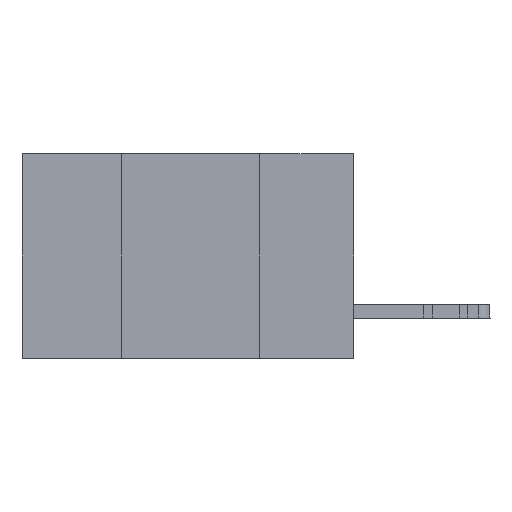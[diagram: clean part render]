
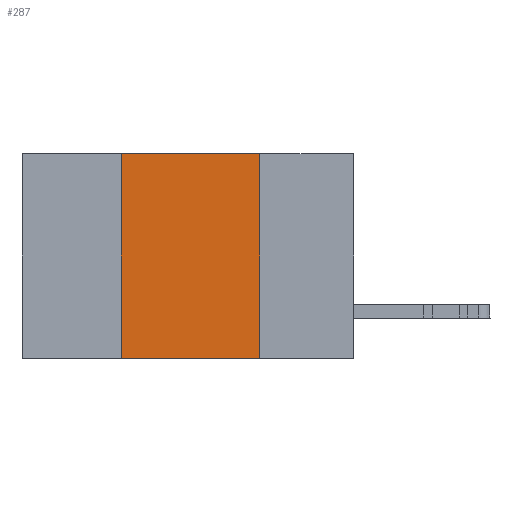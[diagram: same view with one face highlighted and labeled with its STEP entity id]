
A CAD part, left-side view. The second image highlights one B-rep face of the part: STEP entity #287.
In plain terms, the highlighted planar face has unit normal (-1, 0, 0).
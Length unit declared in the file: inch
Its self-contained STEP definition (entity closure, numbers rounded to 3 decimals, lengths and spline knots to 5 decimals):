
#287 = ADVANCED_FACE ( 'NONE', ( #25476 ), #39475, .F. ) ;
#1291 = CARTESIAN_POINT ( 'NONE',  ( 0., 0.17, -0.37 ) ) ;
#1420 = CARTESIAN_POINT ( 'NONE',  ( 0., 0.42, 0. ) ) ;
#2200 = ORIENTED_EDGE ( 'NONE', *, *, #44659, .F. ) ;
#3600 = DIRECTION ( 'NONE',  ( 0., -1., 0. ) ) ;
#4391 = VERTEX_POINT ( 'NONE', #1291 ) ;
#4634 = CARTESIAN_POINT ( 'NONE',  ( 0., 0.6, 0. ) ) ;
#5567 = LINE ( 'NONE', #41276, #23708 ) ;
#6389 = VERTEX_POINT ( 'NONE', #1420 ) ;
#7853 = DIRECTION ( 'NONE',  ( 1., 0., 0. ) ) ;
#12699 = AXIS2_PLACEMENT_3D ( 'NONE', #4634, #7853, #29382 ) ;
#13901 = EDGE_CURVE ( 'NONE', #21801, #6389, #26640, .T. ) ;
#17647 = DIRECTION ( 'NONE',  ( 0., 0., -1. ) ) ;
#18106 = VECTOR ( 'NONE', #17647, 39.37008 ) ;
#18553 = LINE ( 'NONE', #32561, #18106 ) ;
#19304 = CARTESIAN_POINT ( 'NONE',  ( 0., 0.42, 0. ) ) ;
#21801 = VERTEX_POINT ( 'NONE', #23723 ) ;
#22687 = VECTOR ( 'NONE', #44273, 39.37008 ) ;
#23708 = VECTOR ( 'NONE', #30759, 39.37008 ) ;
#23723 = CARTESIAN_POINT ( 'NONE',  ( 0., 0.42, -0.37 ) ) ;
#25476 = FACE_OUTER_BOUND ( 'NONE', #41264, .T. ) ;
#25695 = VERTEX_POINT ( 'NONE', #37241 ) ;
#26640 = LINE ( 'NONE', #19304, #22687 ) ;
#26946 = ORIENTED_EDGE ( 'NONE', *, *, #34697, .F. ) ;
#27190 = ORIENTED_EDGE ( 'NONE', *, *, #13901, .F. ) ;
#29382 = DIRECTION ( 'NONE',  ( 0., 0., -1. ) ) ;
#30759 = DIRECTION ( 'NONE',  ( 0., -1., 0. ) ) ;
#32412 = ORIENTED_EDGE ( 'NONE', *, *, #37601, .T. ) ;
#32561 = CARTESIAN_POINT ( 'NONE',  ( 0., 0.17, 0. ) ) ;
#34697 = EDGE_CURVE ( 'NONE', #6389, #25695, #41851, .T. ) ;
#34770 = CARTESIAN_POINT ( 'NONE',  ( 0., 0.6, 0. ) ) ;
#37241 = CARTESIAN_POINT ( 'NONE',  ( 0., 0.17, 0. ) ) ;
#37601 = EDGE_CURVE ( 'NONE', #21801, #4391, #5567, .T. ) ;
#39475 = PLANE ( 'NONE',  #12699 ) ;
#41176 = VECTOR ( 'NONE', #3600, 39.37008 ) ;
#41264 = EDGE_LOOP ( 'NONE', ( #2200, #26946, #27190, #32412 ) ) ;
#41276 = CARTESIAN_POINT ( 'NONE',  ( 0., 0.6, -0.37 ) ) ;
#41851 = LINE ( 'NONE', #34770, #41176 ) ;
#44273 = DIRECTION ( 'NONE',  ( 0., 0., 1. ) ) ;
#44659 = EDGE_CURVE ( 'NONE', #25695, #4391, #18553, .T. ) ;
